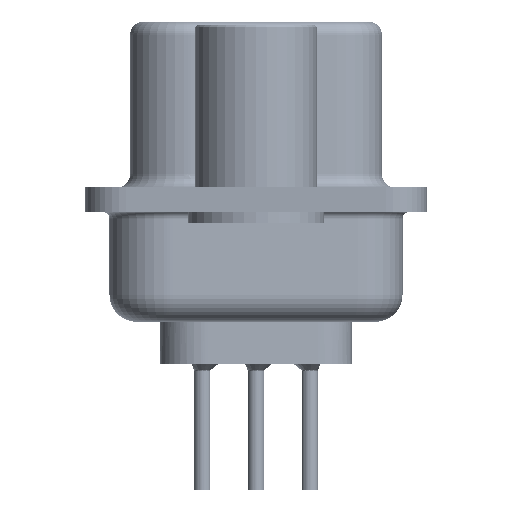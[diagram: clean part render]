
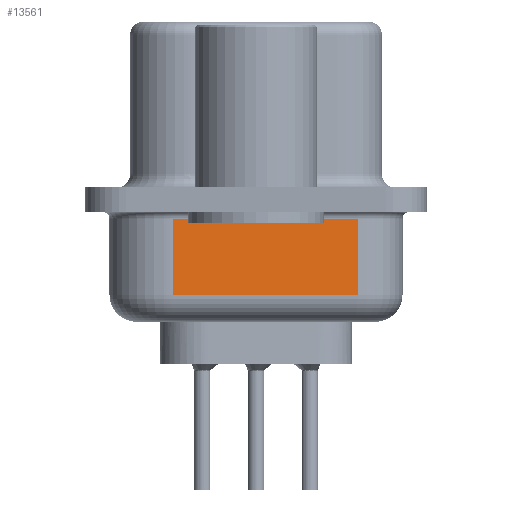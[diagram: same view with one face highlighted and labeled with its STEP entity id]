
A CAD part, left-side view. The second image highlights one B-rep face of the part: STEP entity #13561.
In plain terms, the highlighted planar face has unit normal (-0.985, -0.174, 0).
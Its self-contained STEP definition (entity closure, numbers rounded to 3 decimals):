
#648 = DIRECTION ( 'NONE',  ( 0., 0., 1. ) ) ;
#1068 = FACE_OUTER_BOUND ( 'NONE', #34207, .T. ) ;
#1713 = DIRECTION ( 'NONE',  ( -0.174, 0.985, 0. ) ) ;
#1918 = EDGE_CURVE ( 'NONE', #2711, #11995, #13758, .T. ) ;
#2170 = LINE ( 'NONE', #30904, #17996 ) ;
#2711 = VERTEX_POINT ( 'NONE', #29260 ) ;
#3318 = DIRECTION ( 'NONE',  ( -0.174, 0.985, 0. ) ) ;
#3566 = VECTOR ( 'NONE', #18428, 1000. ) ;
#4579 = DIRECTION ( 'NONE',  ( 0.174, -0.985, 0. ) ) ;
#5118 = CARTESIAN_POINT ( 'NONE',  ( 3., 3.053, -4.5 ) ) ;
#5384 = ORIENTED_EDGE ( 'NONE', *, *, #12355, .T. ) ;
#8879 = VERTEX_POINT ( 'NONE', #14933 ) ;
#11946 = CARTESIAN_POINT ( 'NONE',  ( 4.199, -3.747, -3.5 ) ) ;
#11995 = VERTEX_POINT ( 'NONE', #12422 ) ;
#12355 = EDGE_CURVE ( 'NONE', #15018, #8879, #16556, .T. ) ;
#12422 = CARTESIAN_POINT ( 'NONE',  ( 3., 3.053, -0.7 ) ) ;
#13561 = ADVANCED_FACE ( 'NONE', ( #1068 ), #29956, .F. ) ;
#13758 = LINE ( 'NONE', #5118, #3566 ) ;
#14933 = CARTESIAN_POINT ( 'NONE',  ( 4.199, -3.747, -0.7 ) ) ;
#15018 = VERTEX_POINT ( 'NONE', #11946 ) ;
#15414 = AXIS2_PLACEMENT_3D ( 'NONE', #24928, #16282, #3318 ) ;
#16282 = DIRECTION ( 'NONE',  ( 0.985, 0.174, 0. ) ) ;
#16556 = LINE ( 'NONE', #19319, #29718 ) ;
#16823 = EDGE_CURVE ( 'NONE', #8879, #11995, #25580, .T. ) ;
#17996 = VECTOR ( 'NONE', #4579, 1000. ) ;
#18045 = ORIENTED_EDGE ( 'NONE', *, *, #1918, .F. ) ;
#18428 = DIRECTION ( 'NONE',  ( 0., 0., 1. ) ) ;
#19319 = CARTESIAN_POINT ( 'NONE',  ( 4.199, -3.747, -4.5 ) ) ;
#20084 = EDGE_CURVE ( 'NONE', #2711, #15018, #2170, .T. ) ;
#23161 = CARTESIAN_POINT ( 'NONE',  ( 3., 3.053, -0.7 ) ) ;
#23938 = VECTOR ( 'NONE', #1713, 1000. ) ;
#24334 = ORIENTED_EDGE ( 'NONE', *, *, #16823, .T. ) ;
#24928 = CARTESIAN_POINT ( 'NONE',  ( 3., 3.053, -4.5 ) ) ;
#25580 = LINE ( 'NONE', #23161, #23938 ) ;
#27061 = ORIENTED_EDGE ( 'NONE', *, *, #20084, .T. ) ;
#29260 = CARTESIAN_POINT ( 'NONE',  ( 3., 3.053, -3.5 ) ) ;
#29718 = VECTOR ( 'NONE', #648, 1000. ) ;
#29956 = PLANE ( 'NONE',  #15414 ) ;
#30904 = CARTESIAN_POINT ( 'NONE',  ( 3., 3.053, -3.5 ) ) ;
#34207 = EDGE_LOOP ( 'NONE', ( #18045, #27061, #5384, #24334 ) ) ;
